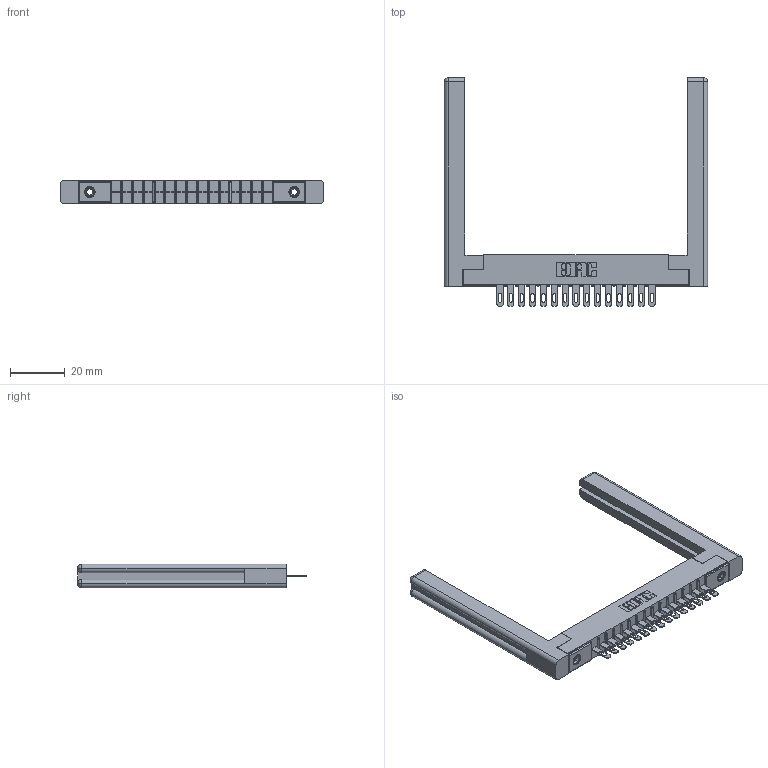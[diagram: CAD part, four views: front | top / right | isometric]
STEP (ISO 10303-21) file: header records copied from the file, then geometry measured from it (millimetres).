
FILE_DESCRIPTION (( 'STEP AP203' ), '1' );
FILE_NAME ('316-015-500-158.STEP', '2018-07-31T00:48:15', ( '' ), ( '' ), 'SwSTEP 2.0', 'SolidWorks 2016', '' );
FILE_SCHEMA (( 'CONFIG_CONTROL_DESIGN' ));
Length unit declared in the file: inch
Products named in the file (5): 307-220-058; 316-015-500-158; 306 Part_.156 Dia; 306-290-001_100; 345-250-001_345-250-001-102
Assembly tree (20 placements, depth 2):
  316-015-500-158
    306 Part_.156 Dia
    306-290-001_100  x15
    345-250-001_345-250-001-102  x2
    307-220-058  x2
Bounding box: 96.06 x 83.52 x 8.71 mm (x, y, z)
Volume: 14237.3 mm3; surface area: 15044.8 mm2
Topology: 20 solids, 20 shells, 1398 faces, 3895 edges, 2502 vertices
Faces by surface type: plane 902, cylinder 412, sphere 60, cone 12, torus 12
Entity records: 20283 total; most frequent: CARTESIAN_POINT 3411, DIRECTION 3322, ORIENTED_EDGE 3320, EDGE_CURVE 1660, LINE 1276, VECTOR 1276, VERTEX_POINT 1058, AXIS2_PLACEMENT_3D 1023
